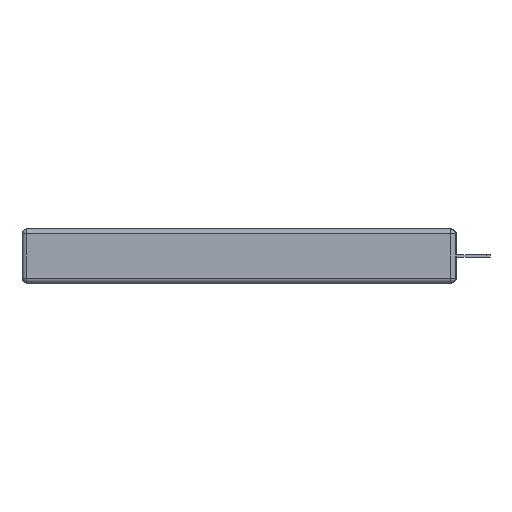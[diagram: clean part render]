
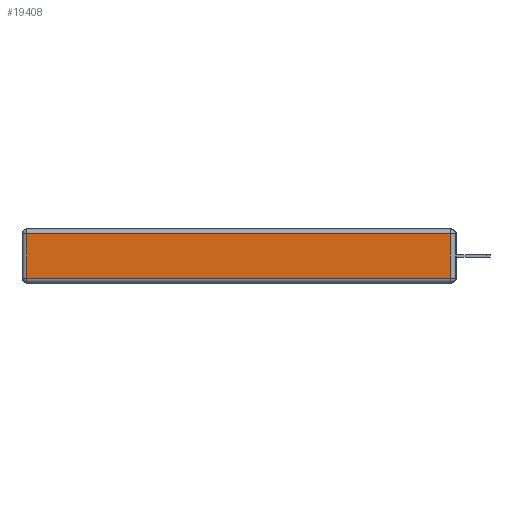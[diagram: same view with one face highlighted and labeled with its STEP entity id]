
A CAD part, left-side view. The second image highlights one B-rep face of the part: STEP entity #19408.
In plain terms, the highlighted planar face has unit normal (-1, 0, 0).
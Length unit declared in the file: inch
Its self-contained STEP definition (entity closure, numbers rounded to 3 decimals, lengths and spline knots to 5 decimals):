
#326 = VERTEX_POINT ( 'NONE', #11671 ) ;
#777 = LINE ( 'NONE', #4660, #16943 ) ;
#851 = VECTOR ( 'NONE', #21459, 39.37008 ) ;
#1182 = LINE ( 'NONE', #14925, #19069 ) ;
#2061 = ORIENTED_EDGE ( 'NONE', *, *, #7437, .T. ) ;
#3239 = DIRECTION ( 'NONE',  ( -1., 0., 0. ) ) ;
#4294 = EDGE_LOOP ( 'NONE', ( #8023, #21556, #2061, #20262 ) ) ;
#4601 = DIRECTION ( 'NONE',  ( 0., -1., 0. ) ) ;
#4660 = CARTESIAN_POINT ( 'NONE',  ( 0., 2.75, -0.03 ) ) ;
#6432 = EDGE_CURVE ( 'NONE', #21887, #326, #1182, .T. ) ;
#7437 = EDGE_CURVE ( 'NONE', #9791, #8439, #777, .T. ) ;
#7624 = CARTESIAN_POINT ( 'NONE',  ( 0., 2.72, -0.03 ) ) ;
#8023 = ORIENTED_EDGE ( 'NONE', *, *, #6432, .T. ) ;
#8039 = EDGE_CURVE ( 'NONE', #326, #9791, #19291, .T. ) ;
#8439 = VERTEX_POINT ( 'NONE', #7624 ) ;
#8531 = CARTESIAN_POINT ( 'NONE',  ( 0., 0.03, -0.03 ) ) ;
#8804 = VECTOR ( 'NONE', #13021, 39.37008 ) ;
#9791 = VERTEX_POINT ( 'NONE', #8531 ) ;
#10479 = CARTESIAN_POINT ( 'NONE',  ( 0., 2.72, -0.313 ) ) ;
#11064 = CARTESIAN_POINT ( 'NONE',  ( 0., 2.72, -0.343 ) ) ;
#11671 = CARTESIAN_POINT ( 'NONE',  ( 0., 0.03, -0.313 ) ) ;
#12290 = PLANE ( 'NONE',  #12533 ) ;
#12533 = AXIS2_PLACEMENT_3D ( 'NONE', #18939, #3239, #19269 ) ;
#13021 = DIRECTION ( 'NONE',  ( 0., 0., -1. ) ) ;
#14137 = CARTESIAN_POINT ( 'NONE',  ( 0., 0.03, -0.343 ) ) ;
#14925 = CARTESIAN_POINT ( 'NONE',  ( 0., 0., -0.313 ) ) ;
#16943 = VECTOR ( 'NONE', #18312, 39.37008 ) ;
#17829 = LINE ( 'NONE', #11064, #8804 ) ;
#18312 = DIRECTION ( 'NONE',  ( 0., 1., 0. ) ) ;
#18575 = EDGE_CURVE ( 'NONE', #8439, #21887, #17829, .T. ) ;
#18939 = CARTESIAN_POINT ( 'NONE',  ( 0., 0., -0.343 ) ) ;
#19069 = VECTOR ( 'NONE', #4601, 39.37008 ) ;
#19269 = DIRECTION ( 'NONE',  ( 0., 0., 1. ) ) ;
#19291 = LINE ( 'NONE', #14137, #851 ) ;
#19408 = ADVANCED_FACE ( 'NONE', ( #20968 ), #12290, .T. ) ;
#20262 = ORIENTED_EDGE ( 'NONE', *, *, #18575, .T. ) ;
#20968 = FACE_OUTER_BOUND ( 'NONE', #4294, .T. ) ;
#21459 = DIRECTION ( 'NONE',  ( 0., 0., 1. ) ) ;
#21556 = ORIENTED_EDGE ( 'NONE', *, *, #8039, .T. ) ;
#21887 = VERTEX_POINT ( 'NONE', #10479 ) ;
